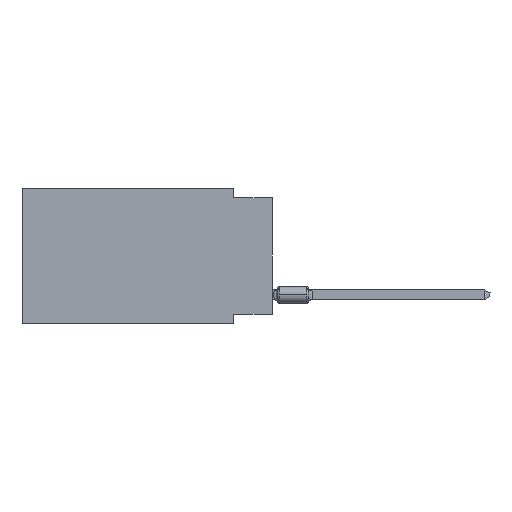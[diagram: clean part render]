
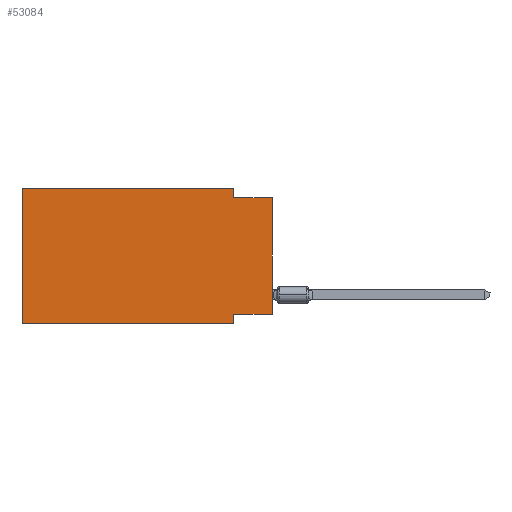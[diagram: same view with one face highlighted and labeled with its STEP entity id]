
A CAD part, left-side view. The second image highlights one B-rep face of the part: STEP entity #53084.
In plain terms, the highlighted planar face has unit normal (-1, 0, 0).
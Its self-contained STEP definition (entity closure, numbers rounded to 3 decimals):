
#2356 = CARTESIAN_POINT ( 'NONE',  ( 0., 2.54, 0. ) ) ;
#3913 = ORIENTED_EDGE ( 'NONE', *, *, #11136, .F. ) ;
#4003 = LINE ( 'NONE', #57517, #102059 ) ;
#5410 = LINE ( 'NONE', #77164, #94905 ) ;
#5531 = VERTEX_POINT ( 'NONE', #2356 ) ;
#7536 = LINE ( 'NONE', #95769, #80592 ) ;
#8856 = AXIS2_PLACEMENT_3D ( 'NONE', #70098, #104788, #78329 ) ;
#11136 = EDGE_CURVE ( 'NONE', #5531, #69469, #4003, .T. ) ;
#15195 = VERTEX_POINT ( 'NONE', #98916 ) ;
#16233 = VECTOR ( 'NONE', #52729, 1000. ) ;
#16921 = DIRECTION ( 'NONE',  ( 0., -1., 0. ) ) ;
#17074 = EDGE_CURVE ( 'NONE', #15195, #79824, #7536, .T. ) ;
#18001 = LINE ( 'NONE', #36238, #16233 ) ;
#19343 = DIRECTION ( 'NONE',  ( 0., -1., 0. ) ) ;
#23835 = ORIENTED_EDGE ( 'NONE', *, *, #104743, .F. ) ;
#24212 = CARTESIAN_POINT ( 'NONE',  ( 0., 2.54, -0.635 ) ) ;
#32030 = CARTESIAN_POINT ( 'NONE',  ( 0., 2.54, -8.89 ) ) ;
#32388 = VECTOR ( 'NONE', #16921, 1000. ) ;
#35054 = CARTESIAN_POINT ( 'NONE',  ( 0., 0., -8.255 ) ) ;
#36238 = CARTESIAN_POINT ( 'NONE',  ( 0., 16.383, 0. ) ) ;
#36870 = ORIENTED_EDGE ( 'NONE', *, *, #113571, .F. ) ;
#42045 = VERTEX_POINT ( 'NONE', #35054 ) ;
#42242 = DIRECTION ( 'NONE',  ( 0., 0., -1. ) ) ;
#45892 = EDGE_CURVE ( 'NONE', #71305, #5531, #82258, .T. ) ;
#46455 = EDGE_LOOP ( 'NONE', ( #73186, #36870, #3913, #77309, #23835, #58462, #78208, #62838 ) ) ;
#51290 = LINE ( 'NONE', #87138, #53525 ) ;
#51703 = CARTESIAN_POINT ( 'NONE',  ( 0., 16.383, 0. ) ) ;
#52729 = DIRECTION ( 'NONE',  ( 0., 0., 1. ) ) ;
#53084 = ADVANCED_FACE ( 'NONE', ( #68347 ), #114782, .F. ) ;
#53525 = VECTOR ( 'NONE', #58962, 1000. ) ;
#53948 = LINE ( 'NONE', #90384, #32388 ) ;
#56598 = CARTESIAN_POINT ( 'NONE',  ( 0., 0., -0.635 ) ) ;
#57517 = CARTESIAN_POINT ( 'NONE',  ( 0., 2.54, 0. ) ) ;
#58462 = ORIENTED_EDGE ( 'NONE', *, *, #93096, .T. ) ;
#58962 = DIRECTION ( 'NONE',  ( 0., -1., 0. ) ) ;
#61038 = CARTESIAN_POINT ( 'NONE',  ( 0., 0., 0. ) ) ;
#62838 = ORIENTED_EDGE ( 'NONE', *, *, #112366, .F. ) ;
#68347 = FACE_OUTER_BOUND ( 'NONE', #46455, .T. ) ;
#68780 = CARTESIAN_POINT ( 'NONE',  ( 0., 16.383, -8.89 ) ) ;
#69469 = VERTEX_POINT ( 'NONE', #24212 ) ;
#70098 = CARTESIAN_POINT ( 'NONE',  ( 0., 16.383, 0. ) ) ;
#71268 = VECTOR ( 'NONE', #19343, 1000. ) ;
#71305 = VERTEX_POINT ( 'NONE', #51703 ) ;
#73186 = ORIENTED_EDGE ( 'NONE', *, *, #85471, .T. ) ;
#77164 = CARTESIAN_POINT ( 'NONE',  ( 0., 0., -8.255 ) ) ;
#77309 = ORIENTED_EDGE ( 'NONE', *, *, #45892, .F. ) ;
#77470 = DIRECTION ( 'NONE',  ( 0., 0., -1. ) ) ;
#77535 = LINE ( 'NONE', #61038, #103305 ) ;
#78208 = ORIENTED_EDGE ( 'NONE', *, *, #17074, .F. ) ;
#78329 = DIRECTION ( 'NONE',  ( 0., 0., -1. ) ) ;
#79824 = VERTEX_POINT ( 'NONE', #32030 ) ;
#80592 = VECTOR ( 'NONE', #42242, 1000. ) ;
#82243 = VERTEX_POINT ( 'NONE', #56598 ) ;
#82258 = LINE ( 'NONE', #91660, #71268 ) ;
#85471 = EDGE_CURVE ( 'NONE', #42045, #82243, #77535, .T. ) ;
#86919 = DIRECTION ( 'NONE',  ( 0., 0., 1. ) ) ;
#87138 = CARTESIAN_POINT ( 'NONE',  ( 0., 0., -0.635 ) ) ;
#90384 = CARTESIAN_POINT ( 'NONE',  ( 0., 16.383, -8.89 ) ) ;
#91660 = CARTESIAN_POINT ( 'NONE',  ( 0., 16.383, 0. ) ) ;
#93096 = EDGE_CURVE ( 'NONE', #97477, #79824, #53948, .T. ) ;
#94905 = VECTOR ( 'NONE', #113038, 1000. ) ;
#95769 = CARTESIAN_POINT ( 'NONE',  ( 0., 2.54, -8.89 ) ) ;
#97477 = VERTEX_POINT ( 'NONE', #68780 ) ;
#98916 = CARTESIAN_POINT ( 'NONE',  ( 0., 2.54, -8.255 ) ) ;
#102059 = VECTOR ( 'NONE', #77470, 1000. ) ;
#103305 = VECTOR ( 'NONE', #86919, 1000. ) ;
#104743 = EDGE_CURVE ( 'NONE', #97477, #71305, #18001, .T. ) ;
#104788 = DIRECTION ( 'NONE',  ( 1., 0., 0. ) ) ;
#112366 = EDGE_CURVE ( 'NONE', #42045, #15195, #5410, .T. ) ;
#113038 = DIRECTION ( 'NONE',  ( 0., 1., 0. ) ) ;
#113571 = EDGE_CURVE ( 'NONE', #69469, #82243, #51290, .T. ) ;
#114782 = PLANE ( 'NONE',  #8856 ) ;
